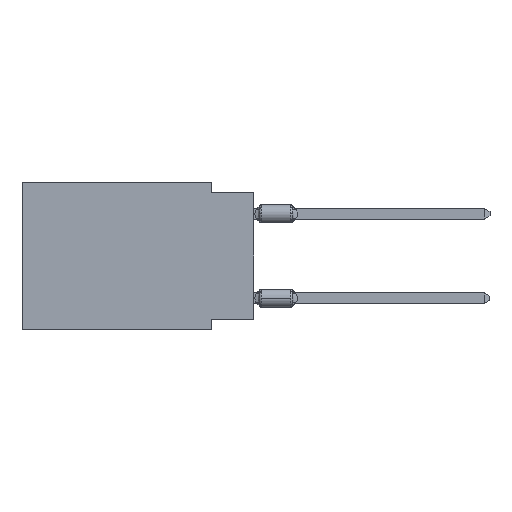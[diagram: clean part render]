
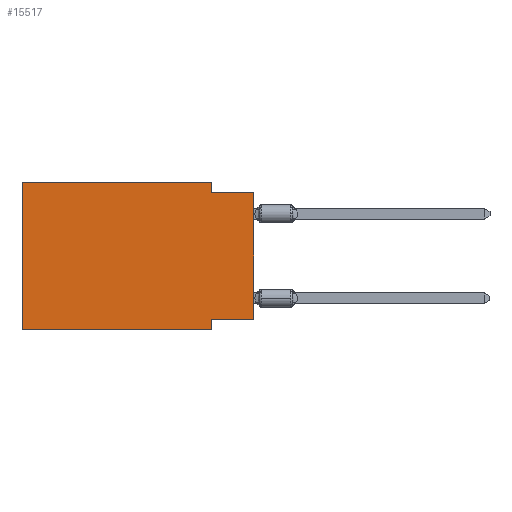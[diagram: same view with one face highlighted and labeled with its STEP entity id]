
A CAD part, left-side view. The second image highlights one B-rep face of the part: STEP entity #15517.
In plain terms, the highlighted planar face has unit normal (-1, 0, 0).
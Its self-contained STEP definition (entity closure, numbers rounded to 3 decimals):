
#67 = AXIS2_PLACEMENT_3D ( 'NONE', #2975, #20715, #15336 ) ;
#160 = EDGE_CURVE ( 'NONE', #12761, #20669, #11586, .T. ) ;
#234 = VECTOR ( 'NONE', #767, 1000. ) ;
#767 = DIRECTION ( 'NONE',  ( 0., 0., 1. ) ) ;
#999 = DIRECTION ( 'NONE',  ( 0., 1., 0. ) ) ;
#1227 = CARTESIAN_POINT ( 'NONE',  ( 0., 0., 0. ) ) ;
#1756 = EDGE_CURVE ( 'NONE', #7024, #20669, #19700, .T. ) ;
#2154 = EDGE_CURVE ( 'NONE', #2708, #13040, #21895, .T. ) ;
#2345 = LINE ( 'NONE', #4090, #9060 ) ;
#2708 = VERTEX_POINT ( 'NONE', #20674 ) ;
#2735 = CARTESIAN_POINT ( 'NONE',  ( 0., 2.54, -8.89 ) ) ;
#2940 = CARTESIAN_POINT ( 'NONE',  ( 0., 0., -0.635 ) ) ;
#2975 = CARTESIAN_POINT ( 'NONE',  ( 0., 13.97, 0. ) ) ;
#3272 = ORIENTED_EDGE ( 'NONE', *, *, #1756, .F. ) ;
#3430 = LINE ( 'NONE', #21177, #13678 ) ;
#3630 = EDGE_CURVE ( 'NONE', #6835, #6272, #3430, .T. ) ;
#3719 = CARTESIAN_POINT ( 'NONE',  ( 0., 0., -0.635 ) ) ;
#4090 = CARTESIAN_POINT ( 'NONE',  ( 0., 13.97, -8.89 ) ) ;
#4226 = DIRECTION ( 'NONE',  ( 0., 0., -1. ) ) ;
#4257 = CARTESIAN_POINT ( 'NONE',  ( 0., 2.54, -8.89 ) ) ;
#5722 = VECTOR ( 'NONE', #4226, 1000. ) ;
#6272 = VERTEX_POINT ( 'NONE', #22591 ) ;
#6489 = DIRECTION ( 'NONE',  ( 0., 0., 1. ) ) ;
#6588 = PLANE ( 'NONE',  #67 ) ;
#6765 = EDGE_LOOP ( 'NONE', ( #20698, #3272, #15361, #9865, #11294, #15467, #21242, #15185 ) ) ;
#6835 = VERTEX_POINT ( 'NONE', #20178 ) ;
#7024 = VERTEX_POINT ( 'NONE', #13739 ) ;
#9048 = VERTEX_POINT ( 'NONE', #22938 ) ;
#9060 = VECTOR ( 'NONE', #11194, 1000. ) ;
#9505 = DIRECTION ( 'NONE',  ( 0., 0., -1. ) ) ;
#9865 = ORIENTED_EDGE ( 'NONE', *, *, #3630, .F. ) ;
#10334 = CARTESIAN_POINT ( 'NONE',  ( 0., 13.97, 0. ) ) ;
#10443 = CARTESIAN_POINT ( 'NONE',  ( 0., 0., -8.255 ) ) ;
#10546 = VECTOR ( 'NONE', #6489, 1000. ) ;
#10816 = DIRECTION ( 'NONE',  ( 0., -1., 0. ) ) ;
#10881 = LINE ( 'NONE', #14721, #5722 ) ;
#11194 = DIRECTION ( 'NONE',  ( 0., -1., 0. ) ) ;
#11294 = ORIENTED_EDGE ( 'NONE', *, *, #11933, .F. ) ;
#11586 = LINE ( 'NONE', #1227, #234 ) ;
#11933 = EDGE_CURVE ( 'NONE', #9048, #6835, #22605, .T. ) ;
#12761 = VERTEX_POINT ( 'NONE', #10443 ) ;
#13040 = VERTEX_POINT ( 'NONE', #2735 ) ;
#13305 = EDGE_CURVE ( 'NONE', #6272, #7024, #10881, .T. ) ;
#13678 = VECTOR ( 'NONE', #22817, 1000. ) ;
#13739 = CARTESIAN_POINT ( 'NONE',  ( 0., 2.54, -0.635 ) ) ;
#13864 = VECTOR ( 'NONE', #999, 1000. ) ;
#14721 = CARTESIAN_POINT ( 'NONE',  ( 0., 2.54, 0. ) ) ;
#15119 = VECTOR ( 'NONE', #9505, 1000. ) ;
#15185 = ORIENTED_EDGE ( 'NONE', *, *, #16836, .F. ) ;
#15336 = DIRECTION ( 'NONE',  ( 0., 0., -1. ) ) ;
#15361 = ORIENTED_EDGE ( 'NONE', *, *, #13305, .F. ) ;
#15467 = ORIENTED_EDGE ( 'NONE', *, *, #17600, .T. ) ;
#15517 = ADVANCED_FACE ( 'NONE', ( #22703 ), #6588, .F. ) ;
#16836 = EDGE_CURVE ( 'NONE', #12761, #2708, #18729, .T. ) ;
#17600 = EDGE_CURVE ( 'NONE', #9048, #13040, #2345, .T. ) ;
#18729 = LINE ( 'NONE', #20369, #13864 ) ;
#19700 = LINE ( 'NONE', #3719, #21475 ) ;
#20178 = CARTESIAN_POINT ( 'NONE',  ( 0., 13.97, 0. ) ) ;
#20369 = CARTESIAN_POINT ( 'NONE',  ( 0., 0., -8.255 ) ) ;
#20669 = VERTEX_POINT ( 'NONE', #2940 ) ;
#20674 = CARTESIAN_POINT ( 'NONE',  ( 0., 2.54, -8.255 ) ) ;
#20698 = ORIENTED_EDGE ( 'NONE', *, *, #160, .T. ) ;
#20715 = DIRECTION ( 'NONE',  ( 1., 0., 0. ) ) ;
#21177 = CARTESIAN_POINT ( 'NONE',  ( 0., 13.97, 0. ) ) ;
#21242 = ORIENTED_EDGE ( 'NONE', *, *, #2154, .F. ) ;
#21475 = VECTOR ( 'NONE', #10816, 1000. ) ;
#21895 = LINE ( 'NONE', #4257, #15119 ) ;
#22591 = CARTESIAN_POINT ( 'NONE',  ( 0., 2.54, 0. ) ) ;
#22605 = LINE ( 'NONE', #10334, #10546 ) ;
#22703 = FACE_OUTER_BOUND ( 'NONE', #6765, .T. ) ;
#22817 = DIRECTION ( 'NONE',  ( 0., -1., 0. ) ) ;
#22938 = CARTESIAN_POINT ( 'NONE',  ( 0., 13.97, -8.89 ) ) ;
